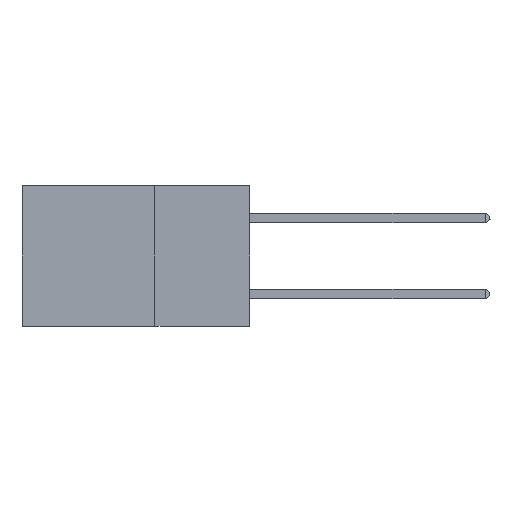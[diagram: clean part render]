
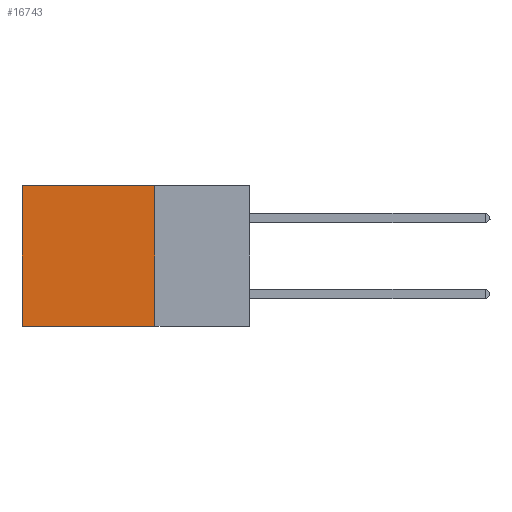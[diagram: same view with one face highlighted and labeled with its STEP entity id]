
A CAD part, left-side view. The second image highlights one B-rep face of the part: STEP entity #16743.
In plain terms, the highlighted planar face has unit normal (-1, 0, 0).
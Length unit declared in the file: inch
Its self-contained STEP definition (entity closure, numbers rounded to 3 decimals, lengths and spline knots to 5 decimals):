
#341 = DIRECTION ( 'NONE',  ( 0., 0., -1. ) ) ;
#383 = DIRECTION ( 'NONE',  ( 0., 1., 0. ) ) ;
#1605 = EDGE_CURVE ( 'NONE', #15033, #19256, #14493, .T. ) ;
#2853 = CARTESIAN_POINT ( 'NONE',  ( 0.2875, 0.25, 0. ) ) ;
#5369 = FACE_OUTER_BOUND ( 'NONE', #30228, .T. ) ;
#7403 = PLANE ( 'NONE',  #28272 ) ;
#9313 = CARTESIAN_POINT ( 'NONE',  ( 0.2875, 0.6, 0. ) ) ;
#9794 = CARTESIAN_POINT ( 'NONE',  ( 0.2875, 0.25, -0.37 ) ) ;
#10164 = CARTESIAN_POINT ( 'NONE',  ( 0.2875, 0.25, -0.37 ) ) ;
#11118 = ORIENTED_EDGE ( 'NONE', *, *, #12025, .F. ) ;
#11699 = DIRECTION ( 'NONE',  ( 0., 0., -1. ) ) ;
#12025 = EDGE_CURVE ( 'NONE', #15783, #19256, #26752, .T. ) ;
#12302 = CARTESIAN_POINT ( 'NONE',  ( 0.2875, 0.6, 0. ) ) ;
#14395 = CARTESIAN_POINT ( 'NONE',  ( 0.2875, 0.25, 0. ) ) ;
#14493 = LINE ( 'NONE', #12302, #15714 ) ;
#14555 = LINE ( 'NONE', #24062, #24466 ) ;
#15033 = VERTEX_POINT ( 'NONE', #9313 ) ;
#15714 = VECTOR ( 'NONE', #11699, 39.37008 ) ;
#15783 = VERTEX_POINT ( 'NONE', #10164 ) ;
#15944 = VERTEX_POINT ( 'NONE', #16526 ) ;
#16526 = CARTESIAN_POINT ( 'NONE',  ( 0.2875, 0.25, 0. ) ) ;
#16743 = ADVANCED_FACE ( 'NONE', ( #5369 ), #7403, .F. ) ;
#19256 = VERTEX_POINT ( 'NONE', #20968 ) ;
#19304 = DIRECTION ( 'NONE',  ( 0., 1., 0. ) ) ;
#19716 = DIRECTION ( 'NONE',  ( 1., 0., 0. ) ) ;
#20079 = VECTOR ( 'NONE', #341, 39.37008 ) ;
#20968 = CARTESIAN_POINT ( 'NONE',  ( 0.2875, 0.6, -0.37 ) ) ;
#21878 = DIRECTION ( 'NONE',  ( 0., 0., -1. ) ) ;
#23466 = EDGE_CURVE ( 'NONE', #15944, #15033, #14555, .T. ) ;
#24062 = CARTESIAN_POINT ( 'NONE',  ( 0.2875, 0.25, 0. ) ) ;
#24466 = VECTOR ( 'NONE', #383, 39.37008 ) ;
#24996 = EDGE_CURVE ( 'NONE', #15944, #15783, #26651, .T. ) ;
#25620 = ORIENTED_EDGE ( 'NONE', *, *, #23466, .T. ) ;
#26651 = LINE ( 'NONE', #2853, #20079 ) ;
#26752 = LINE ( 'NONE', #9794, #26997 ) ;
#26997 = VECTOR ( 'NONE', #19304, 39.37008 ) ;
#27014 = ORIENTED_EDGE ( 'NONE', *, *, #24996, .F. ) ;
#28272 = AXIS2_PLACEMENT_3D ( 'NONE', #14395, #19716, #21878 ) ;
#29198 = ORIENTED_EDGE ( 'NONE', *, *, #1605, .T. ) ;
#30228 = EDGE_LOOP ( 'NONE', ( #29198, #11118, #27014, #25620 ) ) ;
